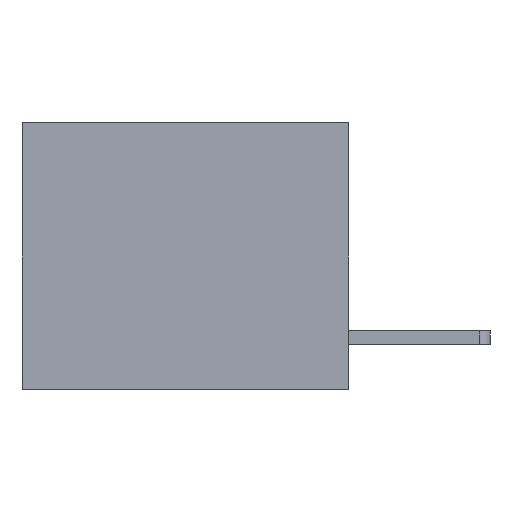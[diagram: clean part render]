
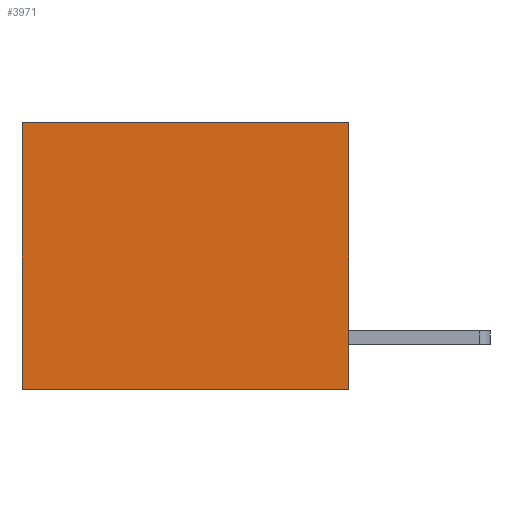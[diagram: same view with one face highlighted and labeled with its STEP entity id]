
A CAD part, left-side view. The second image highlights one B-rep face of the part: STEP entity #3971.
In plain terms, the highlighted planar face has unit normal (-1, 0, 0).
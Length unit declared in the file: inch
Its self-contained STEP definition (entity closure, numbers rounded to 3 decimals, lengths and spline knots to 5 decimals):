
#85 = VERTEX_POINT ( 'NONE', #7037 ) ;
#200 = EDGE_CURVE ( 'NONE', #6593, #9598, #7648, .T. ) ;
#987 = VECTOR ( 'NONE', #7369, 39.37008 ) ;
#1354 = LINE ( 'NONE', #1557, #2120 ) ;
#1557 = CARTESIAN_POINT ( 'NONE',  ( 0.3165, 0., -0.49 ) ) ;
#1716 = ORIENTED_EDGE ( 'NONE', *, *, #3244, .T. ) ;
#1786 = AXIS2_PLACEMENT_3D ( 'NONE', #5513, #7145, #7921 ) ;
#1863 = CARTESIAN_POINT ( 'NONE',  ( 0.3165, 0., -0.49 ) ) ;
#1989 = ORIENTED_EDGE ( 'NONE', *, *, #200, .T. ) ;
#2116 = CARTESIAN_POINT ( 'NONE',  ( 0.3165, 0.6, -0.49 ) ) ;
#2120 = VECTOR ( 'NONE', #7238, 39.37008 ) ;
#2669 = DIRECTION ( 'NONE',  ( 0., 1., 0. ) ) ;
#3244 = EDGE_CURVE ( 'NONE', #9598, #9609, #9664, .T. ) ;
#3971 = ADVANCED_FACE ( 'NONE', ( #6265 ), #9537, .F. ) ;
#4159 = ORIENTED_EDGE ( 'NONE', *, *, #4235, .F. ) ;
#4235 = EDGE_CURVE ( 'NONE', #6593, #85, #1354, .T. ) ;
#4290 = ORIENTED_EDGE ( 'NONE', *, *, #5742, .F. ) ;
#5513 = CARTESIAN_POINT ( 'NONE',  ( 0.3165, 0., -0.49 ) ) ;
#5742 = EDGE_CURVE ( 'NONE', #85, #9609, #9501, .T. ) ;
#5930 = EDGE_LOOP ( 'NONE', ( #1716, #4290, #4159, #1989 ) ) ;
#6047 = CARTESIAN_POINT ( 'NONE',  ( 0.3165, 0.6, -0.49 ) ) ;
#6082 = CARTESIAN_POINT ( 'NONE',  ( 0.3165, 0.6, 0. ) ) ;
#6265 = FACE_OUTER_BOUND ( 'NONE', #5930, .T. ) ;
#6593 = VERTEX_POINT ( 'NONE', #7269 ) ;
#6922 = DIRECTION ( 'NONE',  ( 0., 0., -1. ) ) ;
#7037 = CARTESIAN_POINT ( 'NONE',  ( 0.3165, 0., -0.49 ) ) ;
#7145 = DIRECTION ( 'NONE',  ( 1., 0., 0. ) ) ;
#7238 = DIRECTION ( 'NONE',  ( 0., 0., -1. ) ) ;
#7269 = CARTESIAN_POINT ( 'NONE',  ( 0.3165, 0., 0. ) ) ;
#7369 = DIRECTION ( 'NONE',  ( 0., 1., 0. ) ) ;
#7648 = LINE ( 'NONE', #8917, #987 ) ;
#7921 = DIRECTION ( 'NONE',  ( 0., 0., -1. ) ) ;
#8230 = VECTOR ( 'NONE', #2669, 39.37008 ) ;
#8917 = CARTESIAN_POINT ( 'NONE',  ( 0.3165, 0., 0. ) ) ;
#9501 = LINE ( 'NONE', #1863, #8230 ) ;
#9537 = PLANE ( 'NONE',  #1786 ) ;
#9598 = VERTEX_POINT ( 'NONE', #6082 ) ;
#9609 = VERTEX_POINT ( 'NONE', #6047 ) ;
#9664 = LINE ( 'NONE', #2116, #10169 ) ;
#10169 = VECTOR ( 'NONE', #6922, 39.37008 ) ;
